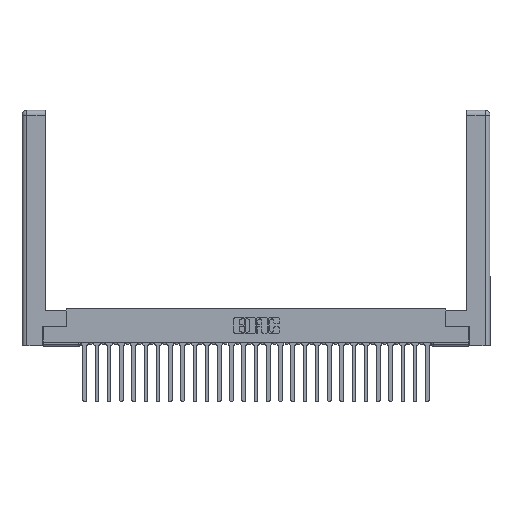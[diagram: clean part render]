
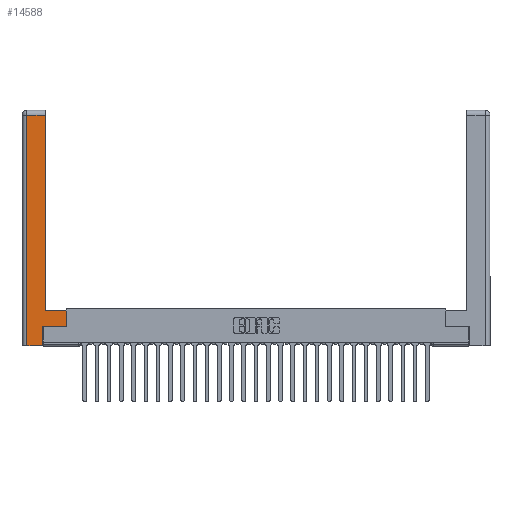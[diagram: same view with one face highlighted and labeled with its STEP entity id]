
A CAD part, top view. The second image highlights one B-rep face of the part: STEP entity #14588.
In plain terms, the highlighted planar face has unit normal (0, 0, 1).
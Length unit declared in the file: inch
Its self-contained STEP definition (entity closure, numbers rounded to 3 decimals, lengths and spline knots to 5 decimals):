
#1757 = DIRECTION ( 'NONE',  ( 0., -1., 0. ) ) ;
#2625 = EDGE_CURVE ( 'NONE', #22825, #6436, #14921, .T. ) ;
#3115 = DIRECTION ( 'NONE',  ( -1., 0., 0. ) ) ;
#3466 = VECTOR ( 'NONE', #14530, 39.37008 ) ;
#3723 = CARTESIAN_POINT ( 'NONE',  ( 0.565, 0.245, 0. ) ) ;
#3914 = ORIENTED_EDGE ( 'NONE', *, *, #12194, .T. ) ;
#4915 = VECTOR ( 'NONE', #17423, 39.37008 ) ;
#5204 = CARTESIAN_POINT ( 'NONE',  ( 0.265, 0., 0. ) ) ;
#5529 = LINE ( 'NONE', #21308, #3466 ) ;
#5621 = VERTEX_POINT ( 'NONE', #14606 ) ;
#6175 = VECTOR ( 'NONE', #1757, 39.37008 ) ;
#6215 = EDGE_CURVE ( 'NONE', #7402, #16013, #13226, .T. ) ;
#6436 = VERTEX_POINT ( 'NONE', #7763 ) ;
#6441 = ORIENTED_EDGE ( 'NONE', *, *, #20020, .T. ) ;
#6527 = CARTESIAN_POINT ( 'NONE',  ( 0.565, 0.45, 0. ) ) ;
#7354 = VECTOR ( 'NONE', #3115, 39.37008 ) ;
#7399 = EDGE_CURVE ( 'NONE', #6436, #19540, #27697, .T. ) ;
#7402 = VERTEX_POINT ( 'NONE', #25336 ) ;
#7444 = ORIENTED_EDGE ( 'NONE', *, *, #19850, .T. ) ;
#7763 = CARTESIAN_POINT ( 'NONE',  ( 0.565, 0.245, 0. ) ) ;
#7802 = DIRECTION ( 'NONE',  ( 0., 1., 0. ) ) ;
#9746 = VECTOR ( 'NONE', #21703, 39.37008 ) ;
#10713 = DIRECTION ( 'NONE',  ( 1., 0., 0. ) ) ;
#11340 = VERTEX_POINT ( 'NONE', #26882 ) ;
#12085 = CARTESIAN_POINT ( 'NONE',  ( 0.565, 0.45, 0. ) ) ;
#12088 = DIRECTION ( 'NONE',  ( -1., 0., 0. ) ) ;
#12194 = EDGE_CURVE ( 'NONE', #11340, #5621, #22563, .T. ) ;
#12935 = CARTESIAN_POINT ( 'NONE',  ( 0.0615, 0., 0. ) ) ;
#13099 = VECTOR ( 'NONE', #15498, 39.37008 ) ;
#13224 = VERTEX_POINT ( 'NONE', #5204 ) ;
#13226 = LINE ( 'NONE', #12935, #6175 ) ;
#14100 = ORIENTED_EDGE ( 'NONE', *, *, #21907, .T. ) ;
#14179 = EDGE_LOOP ( 'NONE', ( #3914, #20146, #22719, #14100, #7444, #22475, #19765, #6441 ) ) ;
#14220 = VECTOR ( 'NONE', #10713, 39.37008 ) ;
#14530 = DIRECTION ( 'NONE',  ( -1., 0., 0. ) ) ;
#14588 = ADVANCED_FACE ( 'NONE', ( #26051 ), #24001, .F. ) ;
#14606 = CARTESIAN_POINT ( 'NONE',  ( 0.295, 2.94, 0. ) ) ;
#14921 = LINE ( 'NONE', #3723, #9746 ) ;
#15498 = DIRECTION ( 'NONE',  ( 0., 1., 0. ) ) ;
#16013 = VERTEX_POINT ( 'NONE', #26232 ) ;
#16677 = CARTESIAN_POINT ( 'NONE',  ( 0.295, 0.45, 0. ) ) ;
#16803 = EDGE_CURVE ( 'NONE', #5621, #7402, #5529, .T. ) ;
#16950 = CARTESIAN_POINT ( 'NONE',  ( 0., 0., 0. ) ) ;
#17005 = AXIS2_PLACEMENT_3D ( 'NONE', #16950, #23427, #12088 ) ;
#17076 = LINE ( 'NONE', #28243, #14220 ) ;
#17138 = CARTESIAN_POINT ( 'NONE',  ( 0.265, 0.245, 0. ) ) ;
#17423 = DIRECTION ( 'NONE',  ( 0., 1., 0. ) ) ;
#18730 = VECTOR ( 'NONE', #7802, 39.37008 ) ;
#19540 = VERTEX_POINT ( 'NONE', #6527 ) ;
#19765 = ORIENTED_EDGE ( 'NONE', *, *, #7399, .T. ) ;
#19850 = EDGE_CURVE ( 'NONE', #13224, #22825, #28307, .T. ) ;
#20020 = EDGE_CURVE ( 'NONE', #19540, #11340, #25480, .T. ) ;
#20146 = ORIENTED_EDGE ( 'NONE', *, *, #16803, .T. ) ;
#21308 = CARTESIAN_POINT ( 'NONE',  ( 0.0615, 2.94, 0. ) ) ;
#21703 = DIRECTION ( 'NONE',  ( 1., 0., 0. ) ) ;
#21907 = EDGE_CURVE ( 'NONE', #16013, #13224, #17076, .T. ) ;
#22475 = ORIENTED_EDGE ( 'NONE', *, *, #2625, .T. ) ;
#22563 = LINE ( 'NONE', #24897, #13099 ) ;
#22719 = ORIENTED_EDGE ( 'NONE', *, *, #6215, .T. ) ;
#22825 = VERTEX_POINT ( 'NONE', #27014 ) ;
#23427 = DIRECTION ( 'NONE',  ( 0., 0., -1. ) ) ;
#24001 = PLANE ( 'NONE',  #17005 ) ;
#24897 = CARTESIAN_POINT ( 'NONE',  ( 0.295, 3., 0. ) ) ;
#25336 = CARTESIAN_POINT ( 'NONE',  ( 0.0615, 2.94, 0. ) ) ;
#25480 = LINE ( 'NONE', #16677, #7354 ) ;
#26051 = FACE_OUTER_BOUND ( 'NONE', #14179, .T. ) ;
#26232 = CARTESIAN_POINT ( 'NONE',  ( 0.0615, 0., 0. ) ) ;
#26882 = CARTESIAN_POINT ( 'NONE',  ( 0.295, 0.45, 0. ) ) ;
#27014 = CARTESIAN_POINT ( 'NONE',  ( 0.265, 0.245, 0. ) ) ;
#27697 = LINE ( 'NONE', #12085, #18730 ) ;
#28243 = CARTESIAN_POINT ( 'NONE',  ( 0.265, 0., 0. ) ) ;
#28307 = LINE ( 'NONE', #17138, #4915 ) ;
